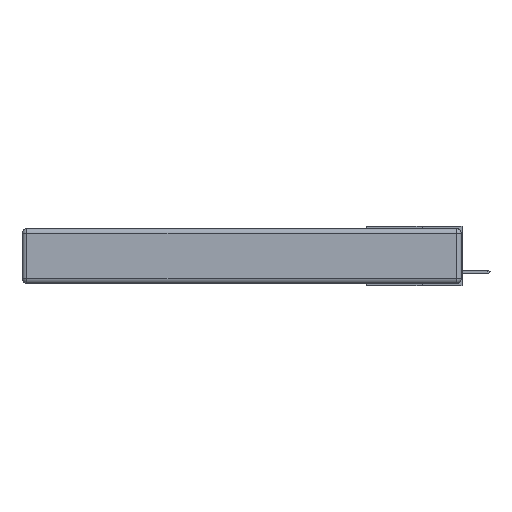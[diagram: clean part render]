
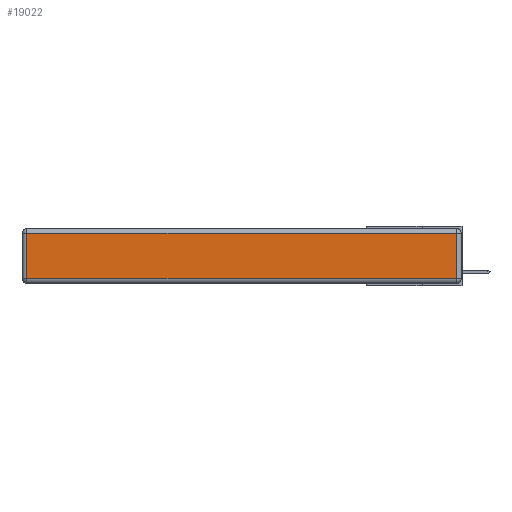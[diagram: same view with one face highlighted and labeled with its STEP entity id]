
A CAD part, left-side view. The second image highlights one B-rep face of the part: STEP entity #19022.
In plain terms, the highlighted planar face has unit normal (-1, 0, 0).
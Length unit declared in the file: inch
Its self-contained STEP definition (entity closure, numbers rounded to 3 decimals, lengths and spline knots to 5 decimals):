
#49 = CARTESIAN_POINT ( 'NONE',  ( 0., 0.03, -0.343 ) ) ;
#881 = LINE ( 'NONE', #6872, #4985 ) ;
#961 = PLANE ( 'NONE',  #11700 ) ;
#1370 = VECTOR ( 'NONE', #23625, 39.37008 ) ;
#3447 = VERTEX_POINT ( 'NONE', #20634 ) ;
#4985 = VECTOR ( 'NONE', #10897, 39.37008 ) ;
#5535 = VECTOR ( 'NONE', #13818, 39.37008 ) ;
#5542 = CARTESIAN_POINT ( 'NONE',  ( 0., 2.75, -0.03 ) ) ;
#6272 = CARTESIAN_POINT ( 'NONE',  ( 0., 0.03, -0.313 ) ) ;
#6725 = DIRECTION ( 'NONE',  ( -1., 0., 0. ) ) ;
#6757 = LINE ( 'NONE', #17655, #1370 ) ;
#6872 = CARTESIAN_POINT ( 'NONE',  ( 0., 2.72, -0.343 ) ) ;
#7999 = LINE ( 'NONE', #49, #11434 ) ;
#8297 = VERTEX_POINT ( 'NONE', #13686 ) ;
#9577 = VERTEX_POINT ( 'NONE', #6272 ) ;
#9893 = DIRECTION ( 'NONE',  ( 0., 0., 1. ) ) ;
#10897 = DIRECTION ( 'NONE',  ( 0., 0., -1. ) ) ;
#11434 = VECTOR ( 'NONE', #9893, 39.37008 ) ;
#11474 = EDGE_CURVE ( 'NONE', #9577, #15939, #7999, .T. ) ;
#11700 = AXIS2_PLACEMENT_3D ( 'NONE', #24842, #6725, #16807 ) ;
#13686 = CARTESIAN_POINT ( 'NONE',  ( 0., 2.72, -0.313 ) ) ;
#13818 = DIRECTION ( 'NONE',  ( 0., 1., 0. ) ) ;
#13959 = FACE_OUTER_BOUND ( 'NONE', #21278, .T. ) ;
#14396 = ORIENTED_EDGE ( 'NONE', *, *, #11474, .T. ) ;
#14703 = EDGE_CURVE ( 'NONE', #3447, #8297, #881, .T. ) ;
#15939 = VERTEX_POINT ( 'NONE', #19410 ) ;
#16018 = EDGE_CURVE ( 'NONE', #15939, #3447, #19667, .T. ) ;
#16807 = DIRECTION ( 'NONE',  ( 0., 0., 1. ) ) ;
#17655 = CARTESIAN_POINT ( 'NONE',  ( 0., 0., -0.313 ) ) ;
#17667 = EDGE_CURVE ( 'NONE', #8297, #9577, #6757, .T. ) ;
#17823 = ORIENTED_EDGE ( 'NONE', *, *, #16018, .T. ) ;
#19022 = ADVANCED_FACE ( 'NONE', ( #13959 ), #961, .T. ) ;
#19410 = CARTESIAN_POINT ( 'NONE',  ( 0., 0.03, -0.03 ) ) ;
#19667 = LINE ( 'NONE', #5542, #5535 ) ;
#20634 = CARTESIAN_POINT ( 'NONE',  ( 0., 2.72, -0.03 ) ) ;
#21278 = EDGE_LOOP ( 'NONE', ( #23146, #14396, #17823, #25227 ) ) ;
#23146 = ORIENTED_EDGE ( 'NONE', *, *, #17667, .T. ) ;
#23625 = DIRECTION ( 'NONE',  ( 0., -1., 0. ) ) ;
#24842 = CARTESIAN_POINT ( 'NONE',  ( 0., 0., -0.343 ) ) ;
#25227 = ORIENTED_EDGE ( 'NONE', *, *, #14703, .T. ) ;
